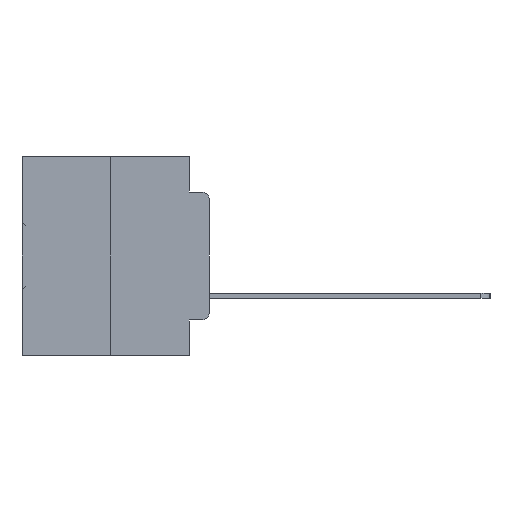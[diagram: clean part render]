
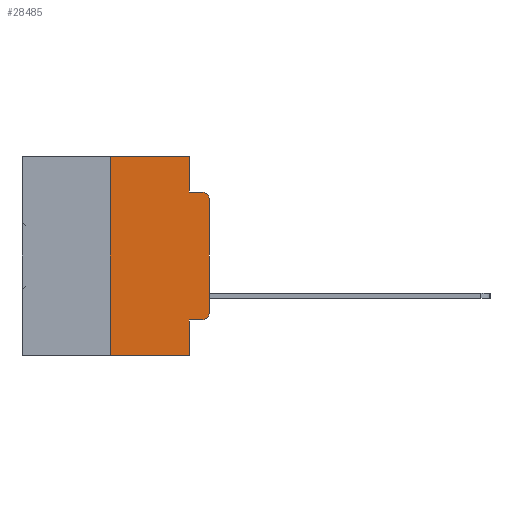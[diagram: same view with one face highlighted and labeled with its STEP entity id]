
A CAD part, left-side view. The second image highlights one B-rep face of the part: STEP entity #28485.
In plain terms, the highlighted planar face has unit normal (-1, 0, 0).
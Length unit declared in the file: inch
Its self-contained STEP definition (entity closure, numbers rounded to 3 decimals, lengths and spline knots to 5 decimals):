
#258 = CARTESIAN_POINT ( 'NONE',  ( 0., 0., -0.3915 ) ) ;
#2269 = EDGE_CURVE ( 'NONE', #12532, #11517, #10845, .T. ) ;
#2593 = PLANE ( 'NONE',  #2733 ) ;
#2659 = VECTOR ( 'NONE', #7178, 39.37008 ) ;
#2733 = AXIS2_PLACEMENT_3D ( 'NONE', #7866, #21018, #5309 ) ;
#2919 = VERTEX_POINT ( 'NONE', #9289 ) ;
#3067 = EDGE_CURVE ( 'NONE', #2919, #25897, #31330, .T. ) ;
#3336 = DIRECTION ( 'NONE',  ( -1., 0., 0. ) ) ;
#3941 = EDGE_CURVE ( 'NONE', #11517, #12907, #20087, .T. ) ;
#3973 = VECTOR ( 'NONE', #23966, 39.37008 ) ;
#4073 = ORIENTED_EDGE ( 'NONE', *, *, #20447, .F. ) ;
#4294 = LINE ( 'NONE', #25505, #31119 ) ;
#4626 = EDGE_CURVE ( 'NONE', #26297, #33225, #11085, .T. ) ;
#5309 = DIRECTION ( 'NONE',  ( 0., 0., -1. ) ) ;
#5949 = CARTESIAN_POINT ( 'NONE',  ( 0., 0.051, -0.5 ) ) ;
#6063 = CARTESIAN_POINT ( 'NONE',  ( 0., 0., -0.1085 ) ) ;
#6165 = ORIENTED_EDGE ( 'NONE', *, *, #4626, .F. ) ;
#6592 = ORIENTED_EDGE ( 'NONE', *, *, #3067, .T. ) ;
#7178 = DIRECTION ( 'NONE',  ( 0., 0., 1. ) ) ;
#7866 = CARTESIAN_POINT ( 'NONE',  ( 0., 0.473, 0. ) ) ;
#8721 = ORIENTED_EDGE ( 'NONE', *, *, #33584, .T. ) ;
#9094 = CARTESIAN_POINT ( 'NONE',  ( 0., 0.25, -0.5 ) ) ;
#9226 = DIRECTION ( 'NONE',  ( 0., 0., -1. ) ) ;
#9289 = CARTESIAN_POINT ( 'NONE',  ( 0., 0.02, -0.4115 ) ) ;
#9541 = ORIENTED_EDGE ( 'NONE', *, *, #31248, .T. ) ;
#10845 = LINE ( 'NONE', #16786, #29785 ) ;
#11085 = LINE ( 'NONE', #16178, #3973 ) ;
#11517 = VERTEX_POINT ( 'NONE', #23389 ) ;
#12401 = VECTOR ( 'NONE', #31831, 39.37008 ) ;
#12511 = DIRECTION ( 'NONE',  ( 0., -1., 0. ) ) ;
#12532 = VERTEX_POINT ( 'NONE', #9094 ) ;
#12907 = VERTEX_POINT ( 'NONE', #31743 ) ;
#13122 = LINE ( 'NONE', #32302, #26027 ) ;
#14213 = VERTEX_POINT ( 'NONE', #6063 ) ;
#14409 = CARTESIAN_POINT ( 'NONE',  ( 0., 0.02, -0.0885 ) ) ;
#14881 = ORIENTED_EDGE ( 'NONE', *, *, #3941, .F. ) ;
#15480 = CARTESIAN_POINT ( 'NONE',  ( 0., 0.051, -0.0885 ) ) ;
#15550 = DIRECTION ( 'NONE',  ( 0., 0., 1. ) ) ;
#16178 = CARTESIAN_POINT ( 'NONE',  ( 0., 0.051, -0.0885 ) ) ;
#16514 = CARTESIAN_POINT ( 'NONE',  ( 0., 0.051, -0.4115 ) ) ;
#16786 = CARTESIAN_POINT ( 'NONE',  ( 0., 0.25, 0. ) ) ;
#16987 = DIRECTION ( 'NONE',  ( 0., 0., -1. ) ) ;
#17013 = CIRCLE ( 'NONE', #32287, 0.02 ) ;
#18514 = VECTOR ( 'NONE', #9226, 39.37008 ) ;
#19129 = CARTESIAN_POINT ( 'NONE',  ( 0., 0.02, -0.1085 ) ) ;
#19155 = EDGE_CURVE ( 'NONE', #32252, #2919, #23071, .T. ) ;
#20087 = LINE ( 'NONE', #29739, #12401 ) ;
#20136 = DIRECTION ( 'NONE',  ( 0., 0., -1. ) ) ;
#20161 = ORIENTED_EDGE ( 'NONE', *, *, #30573, .T. ) ;
#20447 = EDGE_CURVE ( 'NONE', #32252, #29197, #33702, .T. ) ;
#20724 = CARTESIAN_POINT ( 'NONE',  ( 0., 0.02, -0.3915 ) ) ;
#20880 = DIRECTION ( 'NONE',  ( -1., 0., 0. ) ) ;
#21018 = DIRECTION ( 'NONE',  ( 1., 0., 0. ) ) ;
#21439 = FACE_OUTER_BOUND ( 'NONE', #30356, .T. ) ;
#21728 = DIRECTION ( 'NONE',  ( 0., 0., -1. ) ) ;
#22602 = EDGE_CURVE ( 'NONE', #12907, #26297, #13122, .T. ) ;
#22846 = CARTESIAN_POINT ( 'NONE',  ( 0., 0., 0. ) ) ;
#23071 = LINE ( 'NONE', #16514, #29815 ) ;
#23389 = CARTESIAN_POINT ( 'NONE',  ( 0., 0.25, 0. ) ) ;
#23966 = DIRECTION ( 'NONE',  ( 0., -1., 0. ) ) ;
#25505 = CARTESIAN_POINT ( 'NONE',  ( 0., 0.473, -0.5 ) ) ;
#25897 = VERTEX_POINT ( 'NONE', #258 ) ;
#26027 = VECTOR ( 'NONE', #16987, 39.37008 ) ;
#26297 = VERTEX_POINT ( 'NONE', #15480 ) ;
#27329 = CARTESIAN_POINT ( 'NONE',  ( 0., 0.051, 0. ) ) ;
#27739 = ORIENTED_EDGE ( 'NONE', *, *, #22602, .F. ) ;
#28485 = ADVANCED_FACE ( 'NONE', ( #21439 ), #2593, .F. ) ;
#29197 = VERTEX_POINT ( 'NONE', #5949 ) ;
#29267 = DIRECTION ( 'NONE',  ( 0., -1., 0. ) ) ;
#29301 = ORIENTED_EDGE ( 'NONE', *, *, #2269, .F. ) ;
#29739 = CARTESIAN_POINT ( 'NONE',  ( 0., 0.473, 0. ) ) ;
#29785 = VECTOR ( 'NONE', #15550, 39.37008 ) ;
#29815 = VECTOR ( 'NONE', #29267, 39.37008 ) ;
#30356 = EDGE_LOOP ( 'NONE', ( #20161, #8721, #6165, #27739, #14881, #29301, #9541, #4073, #31703, #6592 ) ) ;
#30573 = EDGE_CURVE ( 'NONE', #25897, #14213, #33156, .T. ) ;
#31119 = VECTOR ( 'NONE', #12511, 39.37008 ) ;
#31248 = EDGE_CURVE ( 'NONE', #12532, #29197, #4294, .T. ) ;
#31330 = CIRCLE ( 'NONE', #32177, 0.02 ) ;
#31703 = ORIENTED_EDGE ( 'NONE', *, *, #19155, .T. ) ;
#31743 = CARTESIAN_POINT ( 'NONE',  ( 0., 0.051, 0. ) ) ;
#31831 = DIRECTION ( 'NONE',  ( 0., -1., 0. ) ) ;
#32177 = AXIS2_PLACEMENT_3D ( 'NONE', #20724, #20880, #20136 ) ;
#32252 = VERTEX_POINT ( 'NONE', #32971 ) ;
#32287 = AXIS2_PLACEMENT_3D ( 'NONE', #19129, #3336, #21728 ) ;
#32302 = CARTESIAN_POINT ( 'NONE',  ( 0., 0.051, 0. ) ) ;
#32971 = CARTESIAN_POINT ( 'NONE',  ( 0., 0.051, -0.4115 ) ) ;
#33156 = LINE ( 'NONE', #22846, #2659 ) ;
#33225 = VERTEX_POINT ( 'NONE', #14409 ) ;
#33584 = EDGE_CURVE ( 'NONE', #14213, #33225, #17013, .T. ) ;
#33702 = LINE ( 'NONE', #27329, #18514 ) ;
